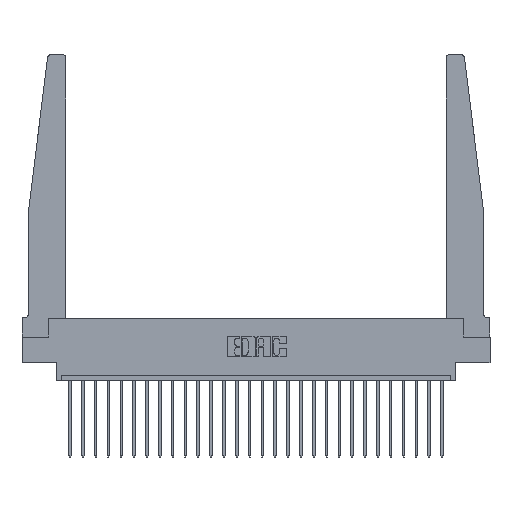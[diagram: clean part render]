
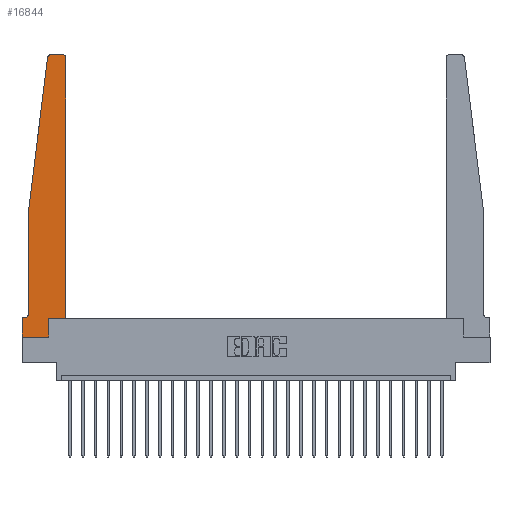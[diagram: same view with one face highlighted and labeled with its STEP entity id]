
A CAD part, top view. The second image highlights one B-rep face of the part: STEP entity #16844.
In plain terms, the highlighted planar face has unit normal (0, 0, 1).
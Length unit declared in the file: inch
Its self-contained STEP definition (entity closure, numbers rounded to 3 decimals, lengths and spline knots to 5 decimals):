
#120 = VERTEX_POINT ( 'NONE', #16857 ) ;
#426 = VERTEX_POINT ( 'NONE', #913 ) ;
#590 = DIRECTION ( 'NONE',  ( 0., 0., -1. ) ) ;
#913 = CARTESIAN_POINT ( 'NONE',  ( 0.2605, 0.18, 0.37 ) ) ;
#1375 = CARTESIAN_POINT ( 'NONE',  ( 0.425, 0.18, 0.37 ) ) ;
#1840 = VERTEX_POINT ( 'NONE', #24380 ) ;
#1868 = CARTESIAN_POINT ( 'NONE',  ( 0.065, 1.25, 0.37 ) ) ;
#1975 = CARTESIAN_POINT ( 'NONE',  ( 0.2605, 0.18, 0.37 ) ) ;
#2023 = AXIS2_PLACEMENT_3D ( 'NONE', #18211, #590, #8642 ) ;
#2163 = CARTESIAN_POINT ( 'NONE',  ( 0.25, 2.75, 0.37 ) ) ;
#2218 = VERTEX_POINT ( 'NONE', #6856 ) ;
#2296 = DIRECTION ( 'NONE',  ( 0., 0., 1. ) ) ;
#2321 = ORIENTED_EDGE ( 'NONE', *, *, #24649, .T. ) ;
#2383 = LINE ( 'NONE', #18305, #16410 ) ;
#2387 = LINE ( 'NONE', #22335, #3396 ) ;
#2682 = CARTESIAN_POINT ( 'NONE',  ( 0., 0.1875, 0.37 ) ) ;
#2791 = VECTOR ( 'NONE', #2938, 39.37008 ) ;
#2938 = DIRECTION ( 'NONE',  ( 0., 1., 0. ) ) ;
#3396 = VECTOR ( 'NONE', #12351, 39.37008 ) ;
#3487 = CARTESIAN_POINT ( 'NONE',  ( 0., 0.1875, 0.37 ) ) ;
#3614 = DIRECTION ( 'NONE',  ( 0., 0., 1. ) ) ;
#3857 = ORIENTED_EDGE ( 'NONE', *, *, #9646, .T. ) ;
#3869 = CARTESIAN_POINT ( 'NONE',  ( 0.065, 1.25, 0.37 ) ) ;
#3870 = CARTESIAN_POINT ( 'NONE',  ( 0.27653, 2.72, 0.37 ) ) ;
#3992 = DIRECTION ( 'NONE',  ( 1., 0., 0. ) ) ;
#3995 = DIRECTION ( 'NONE',  ( -0.122, -0.992, 0. ) ) ;
#4705 = ORIENTED_EDGE ( 'NONE', *, *, #22585, .T. ) ;
#4762 = ORIENTED_EDGE ( 'NONE', *, *, #14683, .T. ) ;
#4841 = DIRECTION ( 'NONE',  ( -1., 0., 0. ) ) ;
#6314 = CARTESIAN_POINT ( 'NONE',  ( 0.395, 2.72, 0.37 ) ) ;
#6550 = ORIENTED_EDGE ( 'NONE', *, *, #9533, .T. ) ;
#6572 = VECTOR ( 'NONE', #24462, 39.37008 ) ;
#6856 = CARTESIAN_POINT ( 'NONE',  ( 0.24675, 2.72367, 0.37 ) ) ;
#8020 = CARTESIAN_POINT ( 'NONE',  ( 0., 0., 0.37 ) ) ;
#8109 = DIRECTION ( 'NONE',  ( 0., -1., 0. ) ) ;
#8270 = VECTOR ( 'NONE', #13333, 39.37008 ) ;
#8642 = DIRECTION ( 'NONE',  ( -1., 0., 0. ) ) ;
#9277 = DIRECTION ( 'NONE',  ( 1., 0., 0. ) ) ;
#9533 = EDGE_CURVE ( 'NONE', #2218, #12373, #17451, .T. ) ;
#9646 = EDGE_CURVE ( 'NONE', #20053, #14728, #23715, .T. ) ;
#9691 = DIRECTION ( 'NONE',  ( 0., 0., 1. ) ) ;
#9948 = LINE ( 'NONE', #8020, #8270 ) ;
#10513 = EDGE_CURVE ( 'NONE', #18260, #426, #25412, .T. ) ;
#12351 = DIRECTION ( 'NONE',  ( -1., 0., 0. ) ) ;
#12373 = VERTEX_POINT ( 'NONE', #1868 ) ;
#12525 = DIRECTION ( 'NONE',  ( 1., 0., 0. ) ) ;
#12890 = CARTESIAN_POINT ( 'NONE',  ( 0., 0., 0.37 ) ) ;
#13274 = VERTEX_POINT ( 'NONE', #24029 ) ;
#13333 = DIRECTION ( 'NONE',  ( 1., 0., 0. ) ) ;
#13595 = CARTESIAN_POINT ( 'NONE',  ( 0.2605, 0., 0.37 ) ) ;
#14318 = ORIENTED_EDGE ( 'NONE', *, *, #17461, .T. ) ;
#14485 = AXIS2_PLACEMENT_3D ( 'NONE', #3870, #3614, #19785 ) ;
#14683 = EDGE_CURVE ( 'NONE', #1840, #20053, #20675, .T. ) ;
#14728 = VERTEX_POINT ( 'NONE', #22624 ) ;
#15295 = AXIS2_PLACEMENT_3D ( 'NONE', #3487, #9691, #3992 ) ;
#15525 = PLANE ( 'NONE',  #15295 ) ;
#15764 = CIRCLE ( 'NONE', #14485, 0.03 ) ;
#16141 = CARTESIAN_POINT ( 'NONE',  ( 0.015, 0.1875, 0.37 ) ) ;
#16291 = LINE ( 'NONE', #16556, #6572 ) ;
#16410 = VECTOR ( 'NONE', #8109, 39.37008 ) ;
#16475 = LINE ( 'NONE', #2163, #18152 ) ;
#16556 = CARTESIAN_POINT ( 'NONE',  ( 0., 0., 0.37 ) ) ;
#16844 = ADVANCED_FACE ( 'NONE', ( #22911 ), #15525, .T. ) ;
#16857 = CARTESIAN_POINT ( 'NONE',  ( 0.27653, 2.75, 0.37 ) ) ;
#16964 = EDGE_CURVE ( 'NONE', #24896, #18260, #9948, .T. ) ;
#17069 = ORIENTED_EDGE ( 'NONE', *, *, #18793, .T. ) ;
#17326 = CIRCLE ( 'NONE', #2023, 0.05 ) ;
#17451 = LINE ( 'NONE', #3869, #19980 ) ;
#17461 = EDGE_CURVE ( 'NONE', #12373, #13274, #2383, .T. ) ;
#17505 = AXIS2_PLACEMENT_3D ( 'NONE', #6314, #2296, #12525 ) ;
#17760 = ORIENTED_EDGE ( 'NONE', *, *, #22853, .T. ) ;
#18072 = CARTESIAN_POINT ( 'NONE',  ( 0.425, 2.72, 0.37 ) ) ;
#18152 = VECTOR ( 'NONE', #4841, 39.37008 ) ;
#18211 = CARTESIAN_POINT ( 'NONE',  ( 0.015, 0.2375, 0.37 ) ) ;
#18260 = VERTEX_POINT ( 'NONE', #13595 ) ;
#18305 = CARTESIAN_POINT ( 'NONE',  ( 0.065, 1.25, 0.37 ) ) ;
#18793 = EDGE_CURVE ( 'NONE', #25553, #22800, #2387, .T. ) ;
#19109 = LINE ( 'NONE', #1375, #19884 ) ;
#19592 = DIRECTION ( 'NONE',  ( 0., 1., 0. ) ) ;
#19601 = ORIENTED_EDGE ( 'NONE', *, *, #25411, .T. ) ;
#19785 = DIRECTION ( 'NONE',  ( 1., 0., 0. ) ) ;
#19884 = VECTOR ( 'NONE', #9277, 39.37008 ) ;
#19980 = VECTOR ( 'NONE', #3995, 39.37008 ) ;
#20053 = VERTEX_POINT ( 'NONE', #18072 ) ;
#20675 = LINE ( 'NONE', #22750, #2791 ) ;
#22335 = CARTESIAN_POINT ( 'NONE',  ( 0.065, 0.1875, 0.37 ) ) ;
#22468 = ORIENTED_EDGE ( 'NONE', *, *, #23334, .T. ) ;
#22585 = EDGE_CURVE ( 'NONE', #22800, #24896, #16291, .T. ) ;
#22624 = CARTESIAN_POINT ( 'NONE',  ( 0.395, 2.75, 0.37 ) ) ;
#22674 = ORIENTED_EDGE ( 'NONE', *, *, #10513, .T. ) ;
#22750 = CARTESIAN_POINT ( 'NONE',  ( 0.425, 0.18, 0.37 ) ) ;
#22800 = VERTEX_POINT ( 'NONE', #2682 ) ;
#22853 = EDGE_CURVE ( 'NONE', #13274, #25553, #17326, .T. ) ;
#22911 = FACE_OUTER_BOUND ( 'NONE', #25097, .T. ) ;
#23334 = EDGE_CURVE ( 'NONE', #14728, #120, #16475, .T. ) ;
#23715 = CIRCLE ( 'NONE', #17505, 0.03 ) ;
#23757 = VECTOR ( 'NONE', #19592, 39.37008 ) ;
#24029 = CARTESIAN_POINT ( 'NONE',  ( 0.065, 0.2375, 0.37 ) ) ;
#24380 = CARTESIAN_POINT ( 'NONE',  ( 0.425, 0.18, 0.37 ) ) ;
#24462 = DIRECTION ( 'NONE',  ( 0., -1., 0. ) ) ;
#24649 = EDGE_CURVE ( 'NONE', #426, #1840, #19109, .T. ) ;
#24896 = VERTEX_POINT ( 'NONE', #12890 ) ;
#25097 = EDGE_LOOP ( 'NONE', ( #22468, #19601, #6550, #14318, #17760, #17069, #4705, #25206, #22674, #2321, #4762, #3857 ) ) ;
#25206 = ORIENTED_EDGE ( 'NONE', *, *, #16964, .T. ) ;
#25411 = EDGE_CURVE ( 'NONE', #120, #2218, #15764, .T. ) ;
#25412 = LINE ( 'NONE', #1975, #23757 ) ;
#25553 = VERTEX_POINT ( 'NONE', #16141 ) ;
